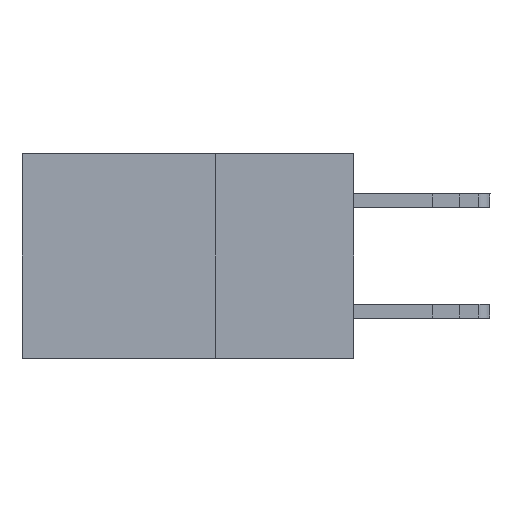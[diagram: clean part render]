
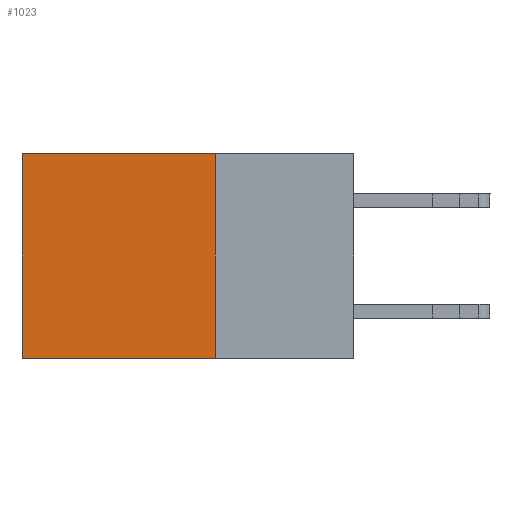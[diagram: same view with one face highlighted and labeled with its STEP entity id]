
A CAD part, left-side view. The second image highlights one B-rep face of the part: STEP entity #1023.
In plain terms, the highlighted planar face has unit normal (-1, 0, 0).
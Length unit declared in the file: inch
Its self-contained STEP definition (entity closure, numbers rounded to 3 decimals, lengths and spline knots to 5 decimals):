
#1023 = ADVANCED_FACE ( 'NONE', ( #9583 ), #16226, .F. ) ;
#2068 = ORIENTED_EDGE ( 'NONE', *, *, #32251, .T. ) ;
#3562 = DIRECTION ( 'NONE',  ( 0., 1., 0. ) ) ;
#4527 = EDGE_LOOP ( 'NONE', ( #6842, #18044, #13128, #2068 ) ) ;
#6109 = VERTEX_POINT ( 'NONE', #11650 ) ;
#6270 = LINE ( 'NONE', #21680, #23913 ) ;
#6451 = VECTOR ( 'NONE', #3562, 39.37008 ) ;
#6681 = LINE ( 'NONE', #28760, #12562 ) ;
#6842 = ORIENTED_EDGE ( 'NONE', *, *, #17046, .T. ) ;
#7224 = VECTOR ( 'NONE', #12699, 39.37008 ) ;
#8097 = VERTEX_POINT ( 'NONE', #19890 ) ;
#9583 = FACE_OUTER_BOUND ( 'NONE', #4527, .T. ) ;
#10199 = EDGE_CURVE ( 'NONE', #8097, #6109, #12771, .T. ) ;
#11650 = CARTESIAN_POINT ( 'NONE',  ( 0.2875, 0.6, -0.37 ) ) ;
#12562 = VECTOR ( 'NONE', #31460, 39.37008 ) ;
#12699 = DIRECTION ( 'NONE',  ( 0., 0., -1. ) ) ;
#12771 = LINE ( 'NONE', #29127, #6451 ) ;
#13122 = CARTESIAN_POINT ( 'NONE',  ( 0.2875, 0.25, 0. ) ) ;
#13128 = ORIENTED_EDGE ( 'NONE', *, *, #13484, .F. ) ;
#13484 = EDGE_CURVE ( 'NONE', #14268, #8097, #28562, .T. ) ;
#13722 = CARTESIAN_POINT ( 'NONE',  ( 0.2875, 0.6, 0. ) ) ;
#14268 = VERTEX_POINT ( 'NONE', #16983 ) ;
#16226 = PLANE ( 'NONE',  #20098 ) ;
#16983 = CARTESIAN_POINT ( 'NONE',  ( 0.2875, 0.25, 0. ) ) ;
#17046 = EDGE_CURVE ( 'NONE', #22374, #6109, #6270, .T. ) ;
#18041 = CARTESIAN_POINT ( 'NONE',  ( 0.2875, 0.25, 0. ) ) ;
#18044 = ORIENTED_EDGE ( 'NONE', *, *, #10199, .F. ) ;
#18647 = DIRECTION ( 'NONE',  ( 0., 0., -1. ) ) ;
#19890 = CARTESIAN_POINT ( 'NONE',  ( 0.2875, 0.25, -0.37 ) ) ;
#20098 = AXIS2_PLACEMENT_3D ( 'NONE', #13122, #21656, #21217 ) ;
#21217 = DIRECTION ( 'NONE',  ( 0., 0., -1. ) ) ;
#21656 = DIRECTION ( 'NONE',  ( 1., 0., 0. ) ) ;
#21680 = CARTESIAN_POINT ( 'NONE',  ( 0.2875, 0.6, 0. ) ) ;
#22374 = VERTEX_POINT ( 'NONE', #13722 ) ;
#23913 = VECTOR ( 'NONE', #18647, 39.37008 ) ;
#28562 = LINE ( 'NONE', #18041, #7224 ) ;
#28760 = CARTESIAN_POINT ( 'NONE',  ( 0.2875, 0.25, 0. ) ) ;
#29127 = CARTESIAN_POINT ( 'NONE',  ( 0.2875, 0.25, -0.37 ) ) ;
#31460 = DIRECTION ( 'NONE',  ( 0., 1., 0. ) ) ;
#32251 = EDGE_CURVE ( 'NONE', #14268, #22374, #6681, .T. ) ;
